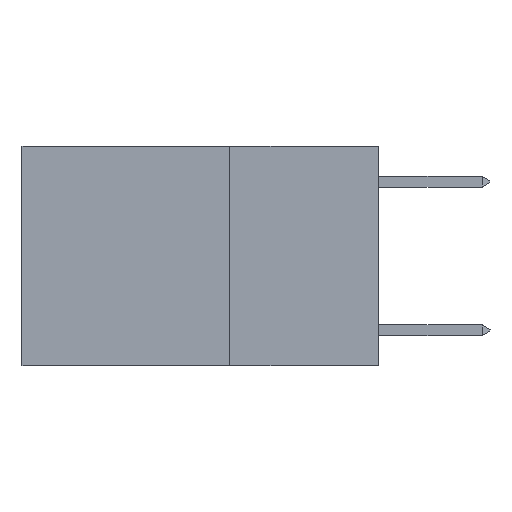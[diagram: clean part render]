
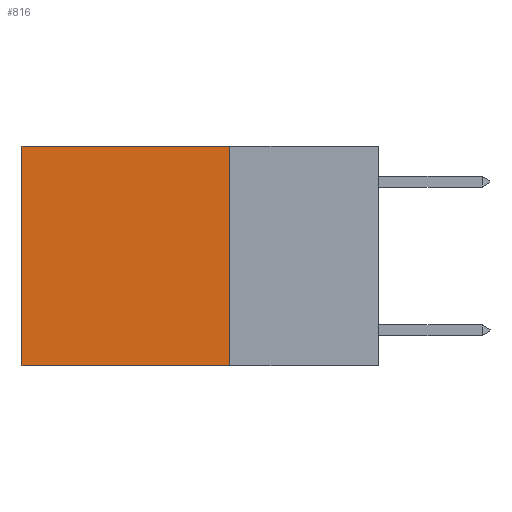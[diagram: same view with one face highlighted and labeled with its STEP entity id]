
A CAD part, left-side view. The second image highlights one B-rep face of the part: STEP entity #816.
In plain terms, the highlighted planar face has unit normal (-1, 0, 0).
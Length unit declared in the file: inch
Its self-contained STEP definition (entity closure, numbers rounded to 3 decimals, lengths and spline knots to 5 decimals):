
#33 = VERTEX_POINT ( 'NONE', #11295 ) ;
#104 = FACE_OUTER_BOUND ( 'NONE', #15798, .T. ) ;
#157 = DIRECTION ( 'NONE',  ( 0., 1., 0. ) ) ;
#816 = ADVANCED_FACE ( 'NONE', ( #104 ), #6674, .F. ) ;
#976 = ORIENTED_EDGE ( 'NONE', *, *, #7776, .F. ) ;
#1611 = VECTOR ( 'NONE', #7555, 39.37008 ) ;
#1911 = ORIENTED_EDGE ( 'NONE', *, *, #16910, .T. ) ;
#3937 = AXIS2_PLACEMENT_3D ( 'NONE', #16438, #17849, #9506 ) ;
#4731 = VERTEX_POINT ( 'NONE', #12164 ) ;
#4996 = EDGE_CURVE ( 'NONE', #15746, #15951, #8373, .T. ) ;
#5289 = CARTESIAN_POINT ( 'NONE',  ( 0.2625, 0.25, -0.37 ) ) ;
#6268 = EDGE_CURVE ( 'NONE', #33, #4731, #15789, .T. ) ;
#6674 = PLANE ( 'NONE',  #3937 ) ;
#7017 = DIRECTION ( 'NONE',  ( 0., 0., -1. ) ) ;
#7089 = CARTESIAN_POINT ( 'NONE',  ( 0.2625, 0.25, 0. ) ) ;
#7431 = CARTESIAN_POINT ( 'NONE',  ( 0.2625, 0.25, 0. ) ) ;
#7555 = DIRECTION ( 'NONE',  ( 0., 1., 0. ) ) ;
#7776 = EDGE_CURVE ( 'NONE', #15951, #4731, #16200, .T. ) ;
#8188 = ORIENTED_EDGE ( 'NONE', *, *, #6268, .T. ) ;
#8370 = VECTOR ( 'NONE', #18064, 39.37008 ) ;
#8373 = LINE ( 'NONE', #7089, #15359 ) ;
#8626 = ORIENTED_EDGE ( 'NONE', *, *, #4996, .F. ) ;
#9506 = DIRECTION ( 'NONE',  ( 0., 0., -1. ) ) ;
#9738 = CARTESIAN_POINT ( 'NONE',  ( 0.2625, 0.6, 0. ) ) ;
#11295 = CARTESIAN_POINT ( 'NONE',  ( 0.2625, 0.6, 0. ) ) ;
#12164 = CARTESIAN_POINT ( 'NONE',  ( 0.2625, 0.6, -0.37 ) ) ;
#14584 = CARTESIAN_POINT ( 'NONE',  ( 0.2625, 0.25, 0. ) ) ;
#15359 = VECTOR ( 'NONE', #7017, 39.37008 ) ;
#15746 = VERTEX_POINT ( 'NONE', #14584 ) ;
#15769 = LINE ( 'NONE', #7431, #17058 ) ;
#15789 = LINE ( 'NONE', #9738, #8370 ) ;
#15798 = EDGE_LOOP ( 'NONE', ( #8188, #976, #8626, #1911 ) ) ;
#15951 = VERTEX_POINT ( 'NONE', #5289 ) ;
#16200 = LINE ( 'NONE', #17291, #1611 ) ;
#16438 = CARTESIAN_POINT ( 'NONE',  ( 0.2625, 0.25, 0. ) ) ;
#16910 = EDGE_CURVE ( 'NONE', #15746, #33, #15769, .T. ) ;
#17058 = VECTOR ( 'NONE', #157, 39.37008 ) ;
#17291 = CARTESIAN_POINT ( 'NONE',  ( 0.2625, 0.25, -0.37 ) ) ;
#17849 = DIRECTION ( 'NONE',  ( 1., 0., 0. ) ) ;
#18064 = DIRECTION ( 'NONE',  ( 0., 0., -1. ) ) ;
